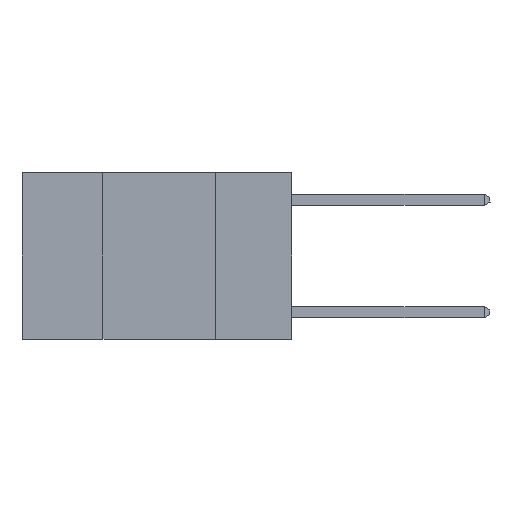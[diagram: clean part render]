
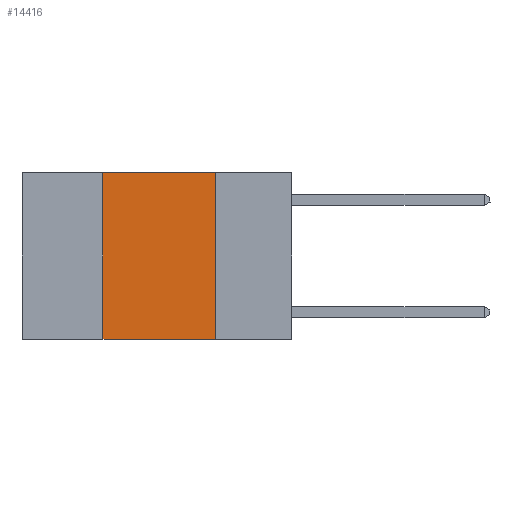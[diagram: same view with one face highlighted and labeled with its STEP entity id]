
A CAD part, left-side view. The second image highlights one B-rep face of the part: STEP entity #14416.
In plain terms, the highlighted planar face has unit normal (-1, 0, 0).
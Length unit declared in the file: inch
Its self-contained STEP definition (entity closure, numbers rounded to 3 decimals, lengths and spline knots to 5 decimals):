
#46 = CARTESIAN_POINT ( 'NONE',  ( 0., 0.17, -0.37 ) ) ;
#165 = EDGE_CURVE ( 'NONE', #11726, #9265, #7292, .T. ) ;
#820 = CARTESIAN_POINT ( 'NONE',  ( 0., 0.6, 0. ) ) ;
#896 = ORIENTED_EDGE ( 'NONE', *, *, #3229, .F. ) ;
#1035 = ORIENTED_EDGE ( 'NONE', *, *, #165, .F. ) ;
#1258 = ORIENTED_EDGE ( 'NONE', *, *, #11183, .F. ) ;
#1658 = ORIENTED_EDGE ( 'NONE', *, *, #16947, .T. ) ;
#3011 = CARTESIAN_POINT ( 'NONE',  ( 0., 0.42, 0. ) ) ;
#3229 = EDGE_CURVE ( 'NONE', #9265, #10468, #10226, .T. ) ;
#5826 = VECTOR ( 'NONE', #13698, 39.37008 ) ;
#6293 = LINE ( 'NONE', #16538, #5826 ) ;
#6320 = CARTESIAN_POINT ( 'NONE',  ( 0., 0.17, 0. ) ) ;
#6838 = DIRECTION ( 'NONE',  ( 1., 0., 0. ) ) ;
#7292 = LINE ( 'NONE', #18372, #18369 ) ;
#8061 = VERTEX_POINT ( 'NONE', #13690 ) ;
#9015 = CARTESIAN_POINT ( 'NONE',  ( 0., 0.17, 0. ) ) ;
#9265 = VERTEX_POINT ( 'NONE', #9015 ) ;
#10226 = LINE ( 'NONE', #6320, #13687 ) ;
#10411 = DIRECTION ( 'NONE',  ( 0., -1., 0. ) ) ;
#10468 = VERTEX_POINT ( 'NONE', #46 ) ;
#10667 = VECTOR ( 'NONE', #10979, 39.37008 ) ;
#10979 = DIRECTION ( 'NONE',  ( 0., -1., 0. ) ) ;
#11183 = EDGE_CURVE ( 'NONE', #8061, #11726, #6293, .T. ) ;
#11726 = VERTEX_POINT ( 'NONE', #3011 ) ;
#13687 = VECTOR ( 'NONE', #13714, 39.37008 ) ;
#13690 = CARTESIAN_POINT ( 'NONE',  ( 0., 0.42, -0.37 ) ) ;
#13698 = DIRECTION ( 'NONE',  ( 0., 0., 1. ) ) ;
#13714 = DIRECTION ( 'NONE',  ( 0., 0., -1. ) ) ;
#14151 = PLANE ( 'NONE',  #18371 ) ;
#14416 = ADVANCED_FACE ( 'NONE', ( #17283 ), #14151, .F. ) ;
#15967 = EDGE_LOOP ( 'NONE', ( #896, #1035, #1258, #1658 ) ) ;
#16538 = CARTESIAN_POINT ( 'NONE',  ( 0., 0.42, 0. ) ) ;
#16947 = EDGE_CURVE ( 'NONE', #8061, #10468, #18304, .T. ) ;
#16977 = DIRECTION ( 'NONE',  ( 0., 0., -1. ) ) ;
#17283 = FACE_OUTER_BOUND ( 'NONE', #15967, .T. ) ;
#18111 = CARTESIAN_POINT ( 'NONE',  ( 0., 0.6, -0.37 ) ) ;
#18304 = LINE ( 'NONE', #18111, #10667 ) ;
#18369 = VECTOR ( 'NONE', #10411, 39.37008 ) ;
#18371 = AXIS2_PLACEMENT_3D ( 'NONE', #820, #6838, #16977 ) ;
#18372 = CARTESIAN_POINT ( 'NONE',  ( 0., 0.6, 0. ) ) ;
